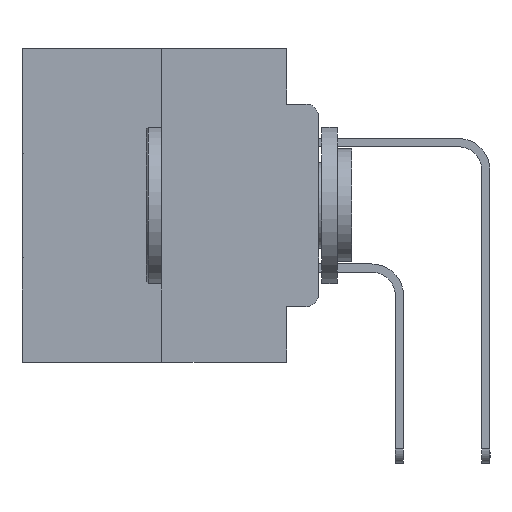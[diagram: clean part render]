
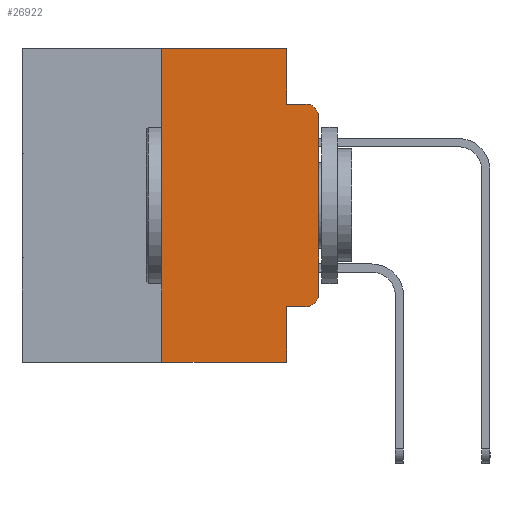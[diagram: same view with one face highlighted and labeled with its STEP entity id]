
A CAD part, left-side view. The second image highlights one B-rep face of the part: STEP entity #26922.
In plain terms, the highlighted planar face has unit normal (-1, 0, 0).
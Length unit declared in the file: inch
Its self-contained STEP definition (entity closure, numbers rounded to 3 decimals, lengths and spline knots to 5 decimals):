
#310 = CARTESIAN_POINT ( 'NONE',  ( 0., 0.051, -0.0885 ) ) ;
#690 = EDGE_CURVE ( 'NONE', #5038, #5309, #25062, .T. ) ;
#990 = LINE ( 'NONE', #10217, #4212 ) ;
#1149 = LINE ( 'NONE', #1301, #29160 ) ;
#1301 = CARTESIAN_POINT ( 'NONE',  ( 0., 0., 0. ) ) ;
#1525 = ORIENTED_EDGE ( 'NONE', *, *, #29275, .F. ) ;
#1702 = ORIENTED_EDGE ( 'NONE', *, *, #29475, .F. ) ;
#1926 = CARTESIAN_POINT ( 'NONE',  ( 0., 0.051, -0.5 ) ) ;
#2591 = CARTESIAN_POINT ( 'NONE',  ( 0., 0.473, 0. ) ) ;
#2927 = ORIENTED_EDGE ( 'NONE', *, *, #25917, .F. ) ;
#3822 = VECTOR ( 'NONE', #4401, 39.37008 ) ;
#4180 = EDGE_CURVE ( 'NONE', #5038, #29105, #7765, .T. ) ;
#4212 = VECTOR ( 'NONE', #14769, 39.37008 ) ;
#4401 = DIRECTION ( 'NONE',  ( 0., -1., 0. ) ) ;
#5038 = VERTEX_POINT ( 'NONE', #25873 ) ;
#5309 = VERTEX_POINT ( 'NONE', #1926 ) ;
#6113 = DIRECTION ( 'NONE',  ( 0., 0., -1. ) ) ;
#6379 = DIRECTION ( 'NONE',  ( -1., 0., 0. ) ) ;
#6414 = LINE ( 'NONE', #15513, #22089 ) ;
#6825 = LINE ( 'NONE', #2591, #3822 ) ;
#7104 = DIRECTION ( 'NONE',  ( 1., 0., 0. ) ) ;
#7765 = LINE ( 'NONE', #21394, #9338 ) ;
#8088 = VERTEX_POINT ( 'NONE', #8836 ) ;
#8491 = ORIENTED_EDGE ( 'NONE', *, *, #14060, .T. ) ;
#8836 = CARTESIAN_POINT ( 'NONE',  ( 0., 0., -0.3915 ) ) ;
#9338 = VECTOR ( 'NONE', #26090, 39.37008 ) ;
#10217 = CARTESIAN_POINT ( 'NONE',  ( 0., 0.473, -0.5 ) ) ;
#10925 = DIRECTION ( 'NONE',  ( 0., 0., -1. ) ) ;
#11223 = LINE ( 'NONE', #29110, #27515 ) ;
#11808 = PLANE ( 'NONE',  #23598 ) ;
#11832 = ORIENTED_EDGE ( 'NONE', *, *, #23323, .F. ) ;
#12316 = CARTESIAN_POINT ( 'NONE',  ( 0., 0.25, -0.5 ) ) ;
#12679 = EDGE_CURVE ( 'NONE', #22728, #26623, #21409, .T. ) ;
#13722 = CARTESIAN_POINT ( 'NONE',  ( 0., 0.051, 0. ) ) ;
#13795 = DIRECTION ( 'NONE',  ( 0., -1., 0. ) ) ;
#14060 = EDGE_CURVE ( 'NONE', #8088, #22728, #1149, .T. ) ;
#14607 = VERTEX_POINT ( 'NONE', #15788 ) ;
#14685 = VERTEX_POINT ( 'NONE', #20765 ) ;
#14769 = DIRECTION ( 'NONE',  ( 0., -1., 0. ) ) ;
#15476 = CARTESIAN_POINT ( 'NONE',  ( 0., 0.02, -0.3915 ) ) ;
#15513 = CARTESIAN_POINT ( 'NONE',  ( 0., 0.051, 0. ) ) ;
#15608 = CARTESIAN_POINT ( 'NONE',  ( 0., 0.051, -0.0885 ) ) ;
#15788 = CARTESIAN_POINT ( 'NONE',  ( 0., 0.25, 0. ) ) ;
#16069 = ORIENTED_EDGE ( 'NONE', *, *, #690, .F. ) ;
#17333 = DIRECTION ( 'NONE',  ( 0., 0., -1. ) ) ;
#18019 = AXIS2_PLACEMENT_3D ( 'NONE', #26276, #19450, #17333 ) ;
#18432 = EDGE_CURVE ( 'NONE', #26179, #5309, #990, .T. ) ;
#18604 = FACE_OUTER_BOUND ( 'NONE', #19624, .T. ) ;
#19090 = CARTESIAN_POINT ( 'NONE',  ( 0., 0.02, -0.0885 ) ) ;
#19104 = ORIENTED_EDGE ( 'NONE', *, *, #26333, .T. ) ;
#19450 = DIRECTION ( 'NONE',  ( -1., 0., 0. ) ) ;
#19624 = EDGE_LOOP ( 'NONE', ( #8491, #25130, #11832, #2927, #1702, #1525, #19680, #16069, #28123, #19104 ) ) ;
#19680 = ORIENTED_EDGE ( 'NONE', *, *, #18432, .T. ) ;
#20765 = CARTESIAN_POINT ( 'NONE',  ( 0., 0.051, 0. ) ) ;
#21394 = CARTESIAN_POINT ( 'NONE',  ( 0., 0.051, -0.4115 ) ) ;
#21409 = CIRCLE ( 'NONE', #18019, 0.02 ) ;
#22089 = VECTOR ( 'NONE', #6113, 39.37008 ) ;
#22728 = VERTEX_POINT ( 'NONE', #26698 ) ;
#22816 = DIRECTION ( 'NONE',  ( 0., 0., -1. ) ) ;
#23323 = EDGE_CURVE ( 'NONE', #23458, #26623, #24679, .T. ) ;
#23458 = VERTEX_POINT ( 'NONE', #310 ) ;
#23580 = AXIS2_PLACEMENT_3D ( 'NONE', #15476, #6379, #10925 ) ;
#23598 = AXIS2_PLACEMENT_3D ( 'NONE', #25124, #7104, #27860 ) ;
#24006 = DIRECTION ( 'NONE',  ( 0., 0., 1. ) ) ;
#24054 = CIRCLE ( 'NONE', #23580, 0.02 ) ;
#24531 = DIRECTION ( 'NONE',  ( 0., 0., 1. ) ) ;
#24679 = LINE ( 'NONE', #15608, #29246 ) ;
#25062 = LINE ( 'NONE', #13722, #25410 ) ;
#25124 = CARTESIAN_POINT ( 'NONE',  ( 0., 0.473, 0. ) ) ;
#25130 = ORIENTED_EDGE ( 'NONE', *, *, #12679, .T. ) ;
#25410 = VECTOR ( 'NONE', #22816, 39.37008 ) ;
#25873 = CARTESIAN_POINT ( 'NONE',  ( 0., 0.051, -0.4115 ) ) ;
#25917 = EDGE_CURVE ( 'NONE', #14685, #23458, #6414, .T. ) ;
#26090 = DIRECTION ( 'NONE',  ( 0., -1., 0. ) ) ;
#26179 = VERTEX_POINT ( 'NONE', #12316 ) ;
#26276 = CARTESIAN_POINT ( 'NONE',  ( 0., 0.02, -0.1085 ) ) ;
#26333 = EDGE_CURVE ( 'NONE', #29105, #8088, #24054, .T. ) ;
#26623 = VERTEX_POINT ( 'NONE', #19090 ) ;
#26698 = CARTESIAN_POINT ( 'NONE',  ( 0., 0., -0.1085 ) ) ;
#26922 = ADVANCED_FACE ( 'NONE', ( #18604 ), #11808, .F. ) ;
#27515 = VECTOR ( 'NONE', #24531, 39.37008 ) ;
#27860 = DIRECTION ( 'NONE',  ( 0., 0., -1. ) ) ;
#28071 = CARTESIAN_POINT ( 'NONE',  ( 0., 0.02, -0.4115 ) ) ;
#28123 = ORIENTED_EDGE ( 'NONE', *, *, #4180, .T. ) ;
#29105 = VERTEX_POINT ( 'NONE', #28071 ) ;
#29110 = CARTESIAN_POINT ( 'NONE',  ( 0., 0.25, 0. ) ) ;
#29160 = VECTOR ( 'NONE', #24006, 39.37008 ) ;
#29246 = VECTOR ( 'NONE', #13795, 39.37008 ) ;
#29275 = EDGE_CURVE ( 'NONE', #26179, #14607, #11223, .T. ) ;
#29475 = EDGE_CURVE ( 'NONE', #14607, #14685, #6825, .T. ) ;
